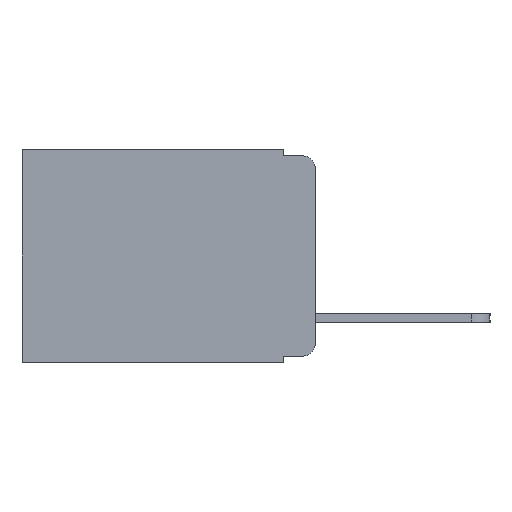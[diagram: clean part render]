
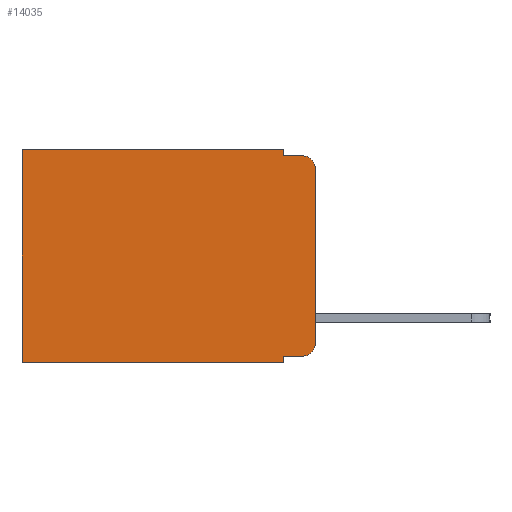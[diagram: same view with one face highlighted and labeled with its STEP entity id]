
A CAD part, left-side view. The second image highlights one B-rep face of the part: STEP entity #14035.
In plain terms, the highlighted planar face has unit normal (-1, 0, 0).
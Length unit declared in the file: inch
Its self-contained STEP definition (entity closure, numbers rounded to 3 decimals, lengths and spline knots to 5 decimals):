
#122 = CARTESIAN_POINT ( 'NONE',  ( 0.298, 0., -0.343 ) ) ;
#153 = DIRECTION ( 'NONE',  ( 1., 0., 0. ) ) ;
#391 = VECTOR ( 'NONE', #5487, 39.37008 ) ;
#738 = ORIENTED_EDGE ( 'NONE', *, *, #21324, .T. ) ;
#1169 = DIRECTION ( 'NONE',  ( 0., -1., 0. ) ) ;
#1462 = CARTESIAN_POINT ( 'NONE',  ( 0.298, 0.02, -0.333 ) ) ;
#1568 = VERTEX_POINT ( 'NONE', #1462 ) ;
#1577 = CARTESIAN_POINT ( 'NONE',  ( 0.298, 0.02, -0.03 ) ) ;
#2060 = EDGE_CURVE ( 'NONE', #15626, #1568, #4953, .T. ) ;
#2137 = CARTESIAN_POINT ( 'NONE',  ( 0.298, 0.051, 0. ) ) ;
#2151 = VECTOR ( 'NONE', #6797, 39.37008 ) ;
#2320 = DIRECTION ( 'NONE',  ( -1., 0., 0. ) ) ;
#2660 = ORIENTED_EDGE ( 'NONE', *, *, #20197, .T. ) ;
#3165 = CARTESIAN_POINT ( 'NONE',  ( 0.298, 0.051, -0.333 ) ) ;
#3212 = ORIENTED_EDGE ( 'NONE', *, *, #3229, .F. ) ;
#3229 = EDGE_CURVE ( 'NONE', #15626, #11082, #4057, .T. ) ;
#3344 = DIRECTION ( 'NONE',  ( 0., 0., -1. ) ) ;
#3399 = CIRCLE ( 'NONE', #5265, 0.02 ) ;
#3713 = CARTESIAN_POINT ( 'NONE',  ( 0.298, 0., 0. ) ) ;
#3885 = DIRECTION ( 'NONE',  ( 0., 0., -1. ) ) ;
#3959 = EDGE_CURVE ( 'NONE', #9228, #4035, #10475, .T. ) ;
#4035 = VERTEX_POINT ( 'NONE', #15653 ) ;
#4057 = LINE ( 'NONE', #9398, #12902 ) ;
#4530 = CARTESIAN_POINT ( 'NONE',  ( 0.298, 0.051, -0.343 ) ) ;
#4953 = LINE ( 'NONE', #11589, #8911 ) ;
#5083 = CARTESIAN_POINT ( 'NONE',  ( 0.298, 0.473, 0. ) ) ;
#5265 = AXIS2_PLACEMENT_3D ( 'NONE', #1577, #13326, #3344 ) ;
#5487 = DIRECTION ( 'NONE',  ( 0., 1., 0. ) ) ;
#5982 = LINE ( 'NONE', #20981, #14202 ) ;
#6321 = EDGE_LOOP ( 'NONE', ( #17971, #9833, #6482, #17487, #738, #16468, #21211, #3212, #7778, #2660 ) ) ;
#6482 = ORIENTED_EDGE ( 'NONE', *, *, #11117, .F. ) ;
#6715 = EDGE_CURVE ( 'NONE', #11400, #8205, #15505, .T. ) ;
#6797 = DIRECTION ( 'NONE',  ( 0., 0., -1. ) ) ;
#7731 = EDGE_CURVE ( 'NONE', #11082, #8205, #10037, .T. ) ;
#7778 = ORIENTED_EDGE ( 'NONE', *, *, #2060, .T. ) ;
#7831 = EDGE_CURVE ( 'NONE', #17514, #16417, #20405, .T. ) ;
#8122 = CARTESIAN_POINT ( 'NONE',  ( 0.298, 0.02, -0.01 ) ) ;
#8205 = VERTEX_POINT ( 'NONE', #15094 ) ;
#8622 = VERTEX_POINT ( 'NONE', #8122 ) ;
#8911 = VECTOR ( 'NONE', #10893, 39.37008 ) ;
#9228 = VERTEX_POINT ( 'NONE', #16358 ) ;
#9336 = CARTESIAN_POINT ( 'NONE',  ( 0.298, 0.051, -0.01 ) ) ;
#9398 = CARTESIAN_POINT ( 'NONE',  ( 0.298, 0.051, 0. ) ) ;
#9833 = ORIENTED_EDGE ( 'NONE', *, *, #13280, .T. ) ;
#9958 = VECTOR ( 'NONE', #12865, 39.37008 ) ;
#10037 = LINE ( 'NONE', #122, #14371 ) ;
#10475 = LINE ( 'NONE', #20641, #9958 ) ;
#10893 = DIRECTION ( 'NONE',  ( 0., -1., 0. ) ) ;
#11082 = VERTEX_POINT ( 'NONE', #4530 ) ;
#11117 = EDGE_CURVE ( 'NONE', #16417, #8622, #5982, .T. ) ;
#11400 = VERTEX_POINT ( 'NONE', #12022 ) ;
#11589 = CARTESIAN_POINT ( 'NONE',  ( 0.298, 0.051, -0.333 ) ) ;
#11810 = VECTOR ( 'NONE', #3885, 39.37008 ) ;
#12022 = CARTESIAN_POINT ( 'NONE',  ( 0.298, 0.473, 0. ) ) ;
#12034 = DIRECTION ( 'NONE',  ( 0., 0., -1. ) ) ;
#12373 = CARTESIAN_POINT ( 'NONE',  ( 0.298, 0.02, -0.313 ) ) ;
#12865 = DIRECTION ( 'NONE',  ( 0., 0., -1. ) ) ;
#12902 = VECTOR ( 'NONE', #18713, 39.37008 ) ;
#13264 = FACE_OUTER_BOUND ( 'NONE', #6321, .T. ) ;
#13280 = EDGE_CURVE ( 'NONE', #9228, #8622, #3399, .T. ) ;
#13326 = DIRECTION ( 'NONE',  ( -1., 0., 0. ) ) ;
#13586 = PLANE ( 'NONE',  #19787 ) ;
#13836 = LINE ( 'NONE', #3713, #391 ) ;
#14024 = DIRECTION ( 'NONE',  ( 0., 0., -1. ) ) ;
#14035 = ADVANCED_FACE ( 'NONE', ( #13264 ), #13586, .F. ) ;
#14202 = VECTOR ( 'NONE', #1169, 39.37008 ) ;
#14371 = VECTOR ( 'NONE', #15251, 39.37008 ) ;
#15094 = CARTESIAN_POINT ( 'NONE',  ( 0.298, 0.473, -0.343 ) ) ;
#15251 = DIRECTION ( 'NONE',  ( 0., 1., 0. ) ) ;
#15505 = LINE ( 'NONE', #5083, #2151 ) ;
#15626 = VERTEX_POINT ( 'NONE', #3165 ) ;
#15653 = CARTESIAN_POINT ( 'NONE',  ( 0.298, 0., -0.313 ) ) ;
#15700 = CIRCLE ( 'NONE', #17765, 0.02 ) ;
#16358 = CARTESIAN_POINT ( 'NONE',  ( 0.298, 0., -0.03 ) ) ;
#16417 = VERTEX_POINT ( 'NONE', #9336 ) ;
#16468 = ORIENTED_EDGE ( 'NONE', *, *, #6715, .T. ) ;
#17487 = ORIENTED_EDGE ( 'NONE', *, *, #7831, .F. ) ;
#17514 = VERTEX_POINT ( 'NONE', #19028 ) ;
#17765 = AXIS2_PLACEMENT_3D ( 'NONE', #12373, #2320, #14024 ) ;
#17971 = ORIENTED_EDGE ( 'NONE', *, *, #3959, .F. ) ;
#18524 = CARTESIAN_POINT ( 'NONE',  ( 0.298, 0., 0. ) ) ;
#18713 = DIRECTION ( 'NONE',  ( 0., 0., -1. ) ) ;
#19028 = CARTESIAN_POINT ( 'NONE',  ( 0.298, 0.051, 0. ) ) ;
#19787 = AXIS2_PLACEMENT_3D ( 'NONE', #18524, #153, #12034 ) ;
#20197 = EDGE_CURVE ( 'NONE', #1568, #4035, #15700, .T. ) ;
#20405 = LINE ( 'NONE', #2137, #11810 ) ;
#20641 = CARTESIAN_POINT ( 'NONE',  ( 0.298, 0., 0. ) ) ;
#20981 = CARTESIAN_POINT ( 'NONE',  ( 0.298, 0.051, -0.01 ) ) ;
#21211 = ORIENTED_EDGE ( 'NONE', *, *, #7731, .F. ) ;
#21324 = EDGE_CURVE ( 'NONE', #17514, #11400, #13836, .T. ) ;
